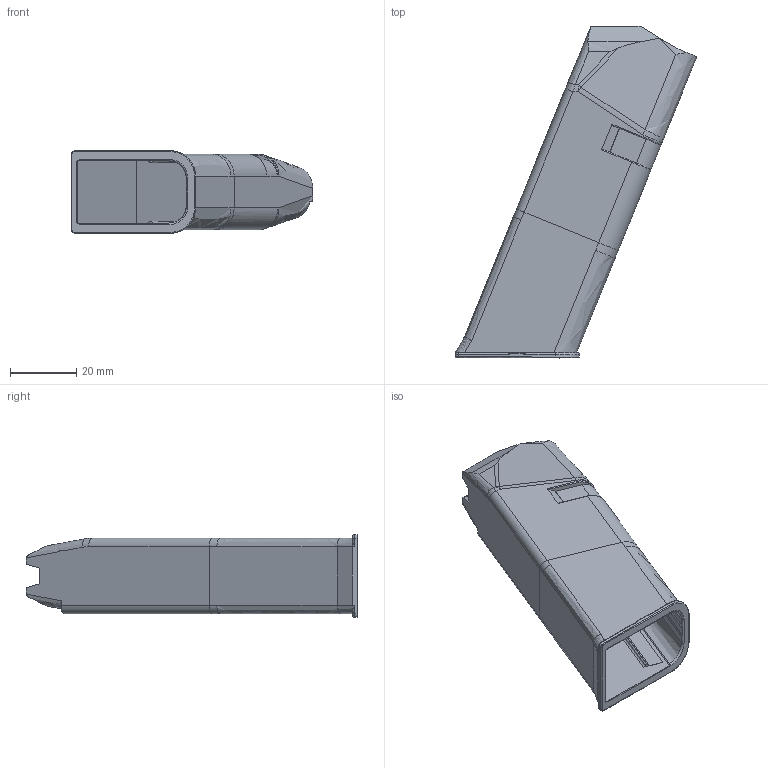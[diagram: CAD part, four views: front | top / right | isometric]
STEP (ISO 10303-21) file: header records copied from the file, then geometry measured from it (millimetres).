
FILE_DESCRIPTION(/* description */ (''),/* implementation_level */ '2;1');
FILE_NAME(/* name */ 'Baby Menenedez Body V1.2.stp',/* time_stamp */ '2019-06-30T13:10:57-05:00',/* author */ ('johne'),/* organization */ (''),/* preprocessor_version */ 'ST-DEVELOPER v16.13',/* originating_system */ 'Autodesk Inventor 2018',/* authorisation */ '');
FILE_SCHEMA (('AUTOMOTIVE_DESIGN { 1 0 10303 214 3 1 1 }'));
Length unit declared in the file: inch
Products named in the file (3): baby menendez; mag bottom; mag top
Assembly tree (2 placements, depth 2):
  baby menendez
    mag bottom
    mag top
Bounding box: 73.04 x 100.3 x 24.87 mm (x, y, z)
Volume: 18082.5 mm3; surface area: 21718.6 mm2
Topology: 4 solids, 6 shells, 443 faces, 1305 edges, 997 vertices
Faces by surface type: plane 250, bspline 135, cylinder 56, cone 2
Entity records: 17327 total; most frequent: CARTESIAN_POINT 6054, ORIENTED_EDGE 2348, DIRECTION 2021, EDGE_CURVE 1173, LINE 759, VECTOR 759, VERTEX_POINT 741, AXIS2_PLACEMENT_3D 631
